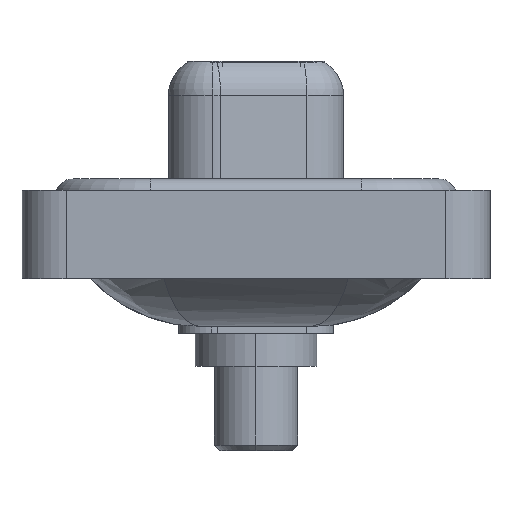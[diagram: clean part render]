
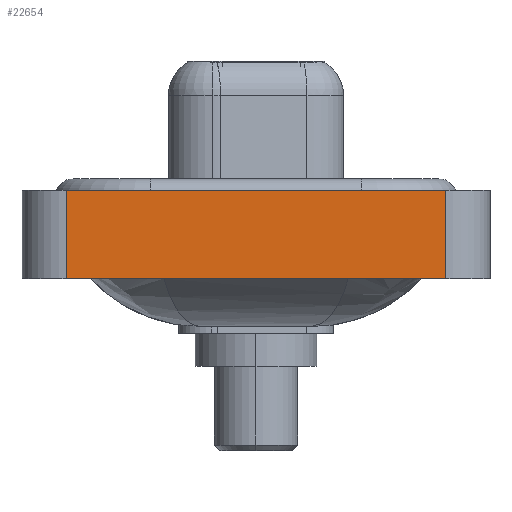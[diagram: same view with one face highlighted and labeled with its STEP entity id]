
A CAD part, left-side view. The second image highlights one B-rep face of the part: STEP entity #22654.
In plain terms, the highlighted planar face has unit normal (-1, 0, 0).
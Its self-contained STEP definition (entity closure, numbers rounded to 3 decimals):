
#99 = ORIENTED_EDGE ( 'NONE', *, *, #10831, .T. ) ;
#1376 = CARTESIAN_POINT ( 'NONE',  ( -7.35, 8.55, -3.6 ) ) ;
#3017 = VECTOR ( 'NONE', #11351, 1000. ) ;
#3241 = CARTESIAN_POINT ( 'NONE',  ( -7.35, -8.55, -3.6 ) ) ;
#3469 = CARTESIAN_POINT ( 'NONE',  ( -7.35, 8.55, -3.6 ) ) ;
#3650 = CARTESIAN_POINT ( 'NONE',  ( -7.35, -8.55, -3.6 ) ) ;
#5310 = PLANE ( 'NONE',  #19517 ) ;
#6007 = CARTESIAN_POINT ( 'NONE',  ( -7.35, -8.55, 0.4 ) ) ;
#7424 = ORIENTED_EDGE ( 'NONE', *, *, #15005, .T. ) ;
#8303 = EDGE_LOOP ( 'NONE', ( #99, #12189, #19318, #7424 ) ) ;
#8904 = CARTESIAN_POINT ( 'NONE',  ( -7.35, -8.55, -3.6 ) ) ;
#9395 = DIRECTION ( 'NONE',  ( -1., 0., 0. ) ) ;
#9467 = DIRECTION ( 'NONE',  ( 0., 0., 1. ) ) ;
#10831 = EDGE_CURVE ( 'NONE', #23129, #10853, #18796, .T. ) ;
#10853 = VERTEX_POINT ( 'NONE', #20731 ) ;
#11351 = DIRECTION ( 'NONE',  ( 0., 0., 1. ) ) ;
#12189 = ORIENTED_EDGE ( 'NONE', *, *, #17383, .F. ) ;
#12815 = DIRECTION ( 'NONE',  ( 0., 0., 1. ) ) ;
#12986 = VECTOR ( 'NONE', #13497, 1000. ) ;
#13497 = DIRECTION ( 'NONE',  ( 0., -1., 0. ) ) ;
#14553 = FACE_OUTER_BOUND ( 'NONE', #8303, .T. ) ;
#15005 = EDGE_CURVE ( 'NONE', #15314, #23129, #16176, .T. ) ;
#15314 = VERTEX_POINT ( 'NONE', #1376 ) ;
#16176 = LINE ( 'NONE', #3241, #19830 ) ;
#17383 = EDGE_CURVE ( 'NONE', #18059, #10853, #21229, .T. ) ;
#18059 = VERTEX_POINT ( 'NONE', #21801 ) ;
#18796 = LINE ( 'NONE', #3650, #24001 ) ;
#19318 = ORIENTED_EDGE ( 'NONE', *, *, #22632, .F. ) ;
#19517 = AXIS2_PLACEMENT_3D ( 'NONE', #8904, #9395, #12815 ) ;
#19830 = VECTOR ( 'NONE', #23626, 1000. ) ;
#20148 = CARTESIAN_POINT ( 'NONE',  ( -7.35, -8.55, -3.6 ) ) ;
#20664 = LINE ( 'NONE', #3469, #3017 ) ;
#20731 = CARTESIAN_POINT ( 'NONE',  ( -7.35, -8.55, 0.4 ) ) ;
#21229 = LINE ( 'NONE', #6007, #12986 ) ;
#21801 = CARTESIAN_POINT ( 'NONE',  ( -7.35, 8.55, 0.4 ) ) ;
#22632 = EDGE_CURVE ( 'NONE', #15314, #18059, #20664, .T. ) ;
#22654 = ADVANCED_FACE ( 'NONE', ( #14553 ), #5310, .T. ) ;
#23129 = VERTEX_POINT ( 'NONE', #20148 ) ;
#23626 = DIRECTION ( 'NONE',  ( 0., -1., 0. ) ) ;
#24001 = VECTOR ( 'NONE', #9467, 1000. ) ;
